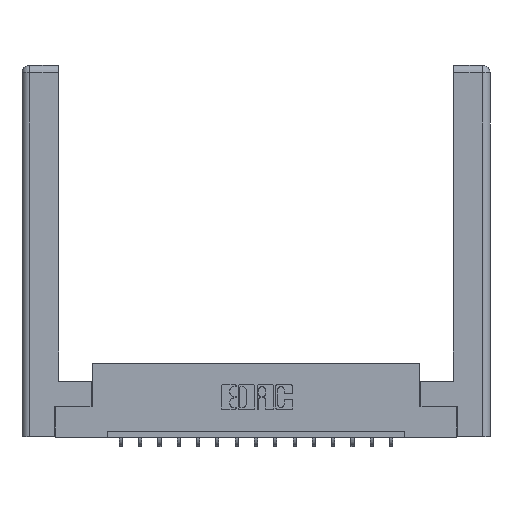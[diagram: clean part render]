
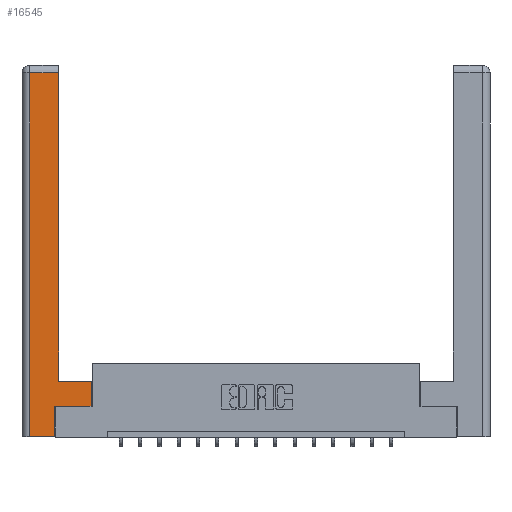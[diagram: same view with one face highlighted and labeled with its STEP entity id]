
A CAD part, top view. The second image highlights one B-rep face of the part: STEP entity #16545.
In plain terms, the highlighted planar face has unit normal (0, 0, 1).
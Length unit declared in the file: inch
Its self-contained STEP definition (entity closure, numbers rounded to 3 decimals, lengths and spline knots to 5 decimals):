
#265 = CARTESIAN_POINT ( 'NONE',  ( 0.0615, 2.94, 0. ) ) ;
#282 = VECTOR ( 'NONE', #7030, 39.37008 ) ;
#493 = DIRECTION ( 'NONE',  ( 0., 1., 0. ) ) ;
#828 = ORIENTED_EDGE ( 'NONE', *, *, #11170, .T. ) ;
#872 = FACE_OUTER_BOUND ( 'NONE', #15116, .T. ) ;
#1794 = VECTOR ( 'NONE', #493, 39.37008 ) ;
#1961 = DIRECTION ( 'NONE',  ( 1., 0., 0. ) ) ;
#2060 = LINE ( 'NONE', #2128, #3752 ) ;
#2128 = CARTESIAN_POINT ( 'NONE',  ( 0.565, 0.245, 0. ) ) ;
#2252 = ORIENTED_EDGE ( 'NONE', *, *, #15856, .T. ) ;
#2704 = ORIENTED_EDGE ( 'NONE', *, *, #17351, .T. ) ;
#2939 = VECTOR ( 'NONE', #9665, 39.37008 ) ;
#3090 = EDGE_CURVE ( 'NONE', #12656, #4626, #9587, .T. ) ;
#3752 = VECTOR ( 'NONE', #1961, 39.37008 ) ;
#3890 = CARTESIAN_POINT ( 'NONE',  ( 0.295, 0.45, 0. ) ) ;
#4164 = VERTEX_POINT ( 'NONE', #15148 ) ;
#4513 = CARTESIAN_POINT ( 'NONE',  ( 0.0615, 2.94, 0. ) ) ;
#4626 = VERTEX_POINT ( 'NONE', #12542 ) ;
#4994 = CARTESIAN_POINT ( 'NONE',  ( 0.265, 0., 0. ) ) ;
#5241 = DIRECTION ( 'NONE',  ( 0., 1., 0. ) ) ;
#5507 = VECTOR ( 'NONE', #5241, 39.37008 ) ;
#5690 = ORIENTED_EDGE ( 'NONE', *, *, #3090, .T. ) ;
#5969 = VERTEX_POINT ( 'NONE', #12724 ) ;
#6026 = VECTOR ( 'NONE', #8900, 39.37008 ) ;
#6149 = PLANE ( 'NONE',  #16349 ) ;
#6507 = LINE ( 'NONE', #15146, #2939 ) ;
#6708 = DIRECTION ( 'NONE',  ( -1., 0., 0. ) ) ;
#7030 = DIRECTION ( 'NONE',  ( -1., 0., 0. ) ) ;
#7103 = EDGE_CURVE ( 'NONE', #5969, #16768, #16675, .T. ) ;
#7345 = CARTESIAN_POINT ( 'NONE',  ( 0.295, 0.45, 0. ) ) ;
#7354 = VERTEX_POINT ( 'NONE', #4994 ) ;
#7503 = ORIENTED_EDGE ( 'NONE', *, *, #9608, .T. ) ;
#7591 = LINE ( 'NONE', #3890, #13686 ) ;
#8243 = ORIENTED_EDGE ( 'NONE', *, *, #7103, .T. ) ;
#8279 = CARTESIAN_POINT ( 'NONE',  ( 0.265, 0., 0. ) ) ;
#8825 = DIRECTION ( 'NONE',  ( 0., 0., -1. ) ) ;
#8900 = DIRECTION ( 'NONE',  ( 0., 1., 0. ) ) ;
#9494 = EDGE_CURVE ( 'NONE', #16768, #12656, #7591, .T. ) ;
#9556 = EDGE_CURVE ( 'NONE', #7354, #4164, #16613, .T. ) ;
#9579 = VERTEX_POINT ( 'NONE', #265 ) ;
#9587 = LINE ( 'NONE', #14236, #6026 ) ;
#9608 = EDGE_CURVE ( 'NONE', #11059, #7354, #15562, .T. ) ;
#9638 = ORIENTED_EDGE ( 'NONE', *, *, #9494, .T. ) ;
#9665 = DIRECTION ( 'NONE',  ( 0., -1., 0. ) ) ;
#9976 = CARTESIAN_POINT ( 'NONE',  ( 0.565, 0.45, 0. ) ) ;
#10298 = DIRECTION ( 'NONE',  ( -1., 0., 0. ) ) ;
#10512 = VECTOR ( 'NONE', #10855, 39.37008 ) ;
#10855 = DIRECTION ( 'NONE',  ( 1., 0., 0. ) ) ;
#11059 = VERTEX_POINT ( 'NONE', #12221 ) ;
#11170 = EDGE_CURVE ( 'NONE', #4164, #5969, #2060, .T. ) ;
#12221 = CARTESIAN_POINT ( 'NONE',  ( 0.0615, 0., 0. ) ) ;
#12542 = CARTESIAN_POINT ( 'NONE',  ( 0.295, 2.94, 0. ) ) ;
#12656 = VERTEX_POINT ( 'NONE', #7345 ) ;
#12724 = CARTESIAN_POINT ( 'NONE',  ( 0.565, 0.245, 0. ) ) ;
#12954 = ORIENTED_EDGE ( 'NONE', *, *, #9556, .T. ) ;
#13686 = VECTOR ( 'NONE', #6708, 39.37008 ) ;
#14236 = CARTESIAN_POINT ( 'NONE',  ( 0.295, 3., 0. ) ) ;
#14277 = CARTESIAN_POINT ( 'NONE',  ( 0., 0., 0. ) ) ;
#15116 = EDGE_LOOP ( 'NONE', ( #5690, #2252, #2704, #7503, #12954, #828, #8243, #9638 ) ) ;
#15146 = CARTESIAN_POINT ( 'NONE',  ( 0.0615, 0., 0. ) ) ;
#15148 = CARTESIAN_POINT ( 'NONE',  ( 0.265, 0.245, 0. ) ) ;
#15260 = CARTESIAN_POINT ( 'NONE',  ( 0.565, 0.45, 0. ) ) ;
#15373 = LINE ( 'NONE', #4513, #282 ) ;
#15562 = LINE ( 'NONE', #8279, #10512 ) ;
#15856 = EDGE_CURVE ( 'NONE', #4626, #9579, #15373, .T. ) ;
#16349 = AXIS2_PLACEMENT_3D ( 'NONE', #14277, #8825, #10298 ) ;
#16545 = ADVANCED_FACE ( 'NONE', ( #872 ), #6149, .F. ) ;
#16613 = LINE ( 'NONE', #17199, #5507 ) ;
#16675 = LINE ( 'NONE', #15260, #1794 ) ;
#16768 = VERTEX_POINT ( 'NONE', #9976 ) ;
#17199 = CARTESIAN_POINT ( 'NONE',  ( 0.265, 0.245, 0. ) ) ;
#17351 = EDGE_CURVE ( 'NONE', #9579, #11059, #6507, .T. ) ;
